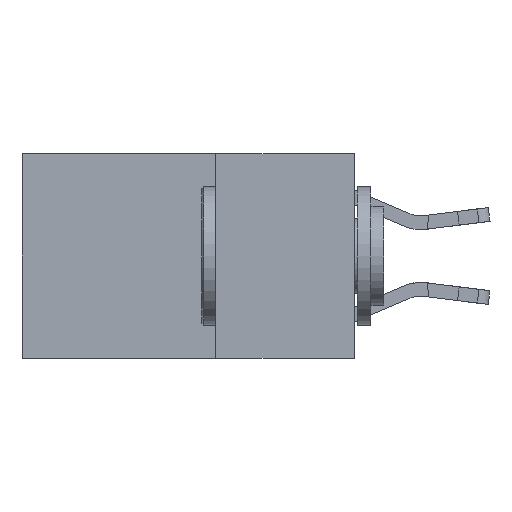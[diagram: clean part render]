
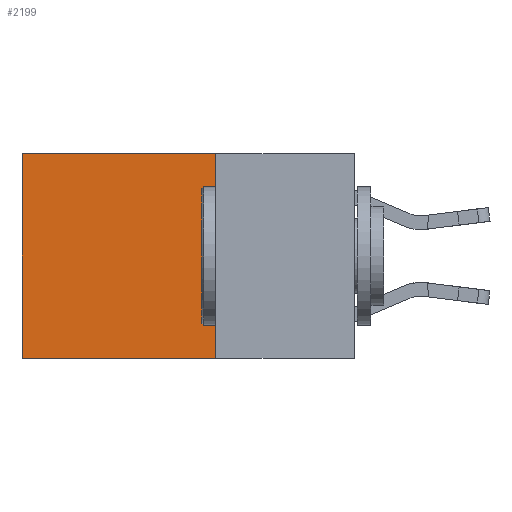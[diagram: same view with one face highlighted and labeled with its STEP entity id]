
A CAD part, left-side view. The second image highlights one B-rep face of the part: STEP entity #2199.
In plain terms, the highlighted planar face has unit normal (-1, 0, 0).
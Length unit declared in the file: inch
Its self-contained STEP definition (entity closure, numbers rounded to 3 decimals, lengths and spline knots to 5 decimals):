
#959 = LINE ( 'NONE', #7559, #9255 ) ;
#967 = EDGE_CURVE ( 'NONE', #9129, #4024, #16546, .T. ) ;
#1625 = VECTOR ( 'NONE', #23283, 39.37008 ) ;
#2199 = ADVANCED_FACE ( 'NONE', ( #18424 ), #14117, .F. ) ;
#2841 = CARTESIAN_POINT ( 'NONE',  ( 0.2625, 0.6, 0. ) ) ;
#4024 = VERTEX_POINT ( 'NONE', #13854 ) ;
#6850 = ORIENTED_EDGE ( 'NONE', *, *, #14675, .T. ) ;
#7559 = CARTESIAN_POINT ( 'NONE',  ( 0.2625, 0.6, 0. ) ) ;
#8101 = VERTEX_POINT ( 'NONE', #17261 ) ;
#9000 = CARTESIAN_POINT ( 'NONE',  ( 0.2625, 0.25, 0. ) ) ;
#9129 = VERTEX_POINT ( 'NONE', #9000 ) ;
#9190 = VERTEX_POINT ( 'NONE', #2841 ) ;
#9255 = VECTOR ( 'NONE', #14155, 39.37008 ) ;
#9317 = EDGE_CURVE ( 'NONE', #9190, #8101, #959, .T. ) ;
#9806 = DIRECTION ( 'NONE',  ( 0., 0., -1. ) ) ;
#10525 = DIRECTION ( 'NONE',  ( 0., 1., 0. ) ) ;
#12370 = ORIENTED_EDGE ( 'NONE', *, *, #967, .F. ) ;
#12374 = ORIENTED_EDGE ( 'NONE', *, *, #24601, .F. ) ;
#13854 = CARTESIAN_POINT ( 'NONE',  ( 0.2625, 0.25, -0.37 ) ) ;
#13942 = CARTESIAN_POINT ( 'NONE',  ( 0.2625, 0.25, -0.37 ) ) ;
#14117 = PLANE ( 'NONE',  #14273 ) ;
#14155 = DIRECTION ( 'NONE',  ( 0., 0., -1. ) ) ;
#14273 = AXIS2_PLACEMENT_3D ( 'NONE', #26725, #18560, #9806 ) ;
#14675 = EDGE_CURVE ( 'NONE', #9129, #9190, #19425, .T. ) ;
#14687 = CARTESIAN_POINT ( 'NONE',  ( 0.2625, 0.25, 0. ) ) ;
#16546 = LINE ( 'NONE', #14687, #1625 ) ;
#16808 = VECTOR ( 'NONE', #10525, 39.37008 ) ;
#17251 = ORIENTED_EDGE ( 'NONE', *, *, #9317, .T. ) ;
#17261 = CARTESIAN_POINT ( 'NONE',  ( 0.2625, 0.6, -0.37 ) ) ;
#18424 = FACE_OUTER_BOUND ( 'NONE', #27170, .T. ) ;
#18560 = DIRECTION ( 'NONE',  ( 1., 0., 0. ) ) ;
#19287 = CARTESIAN_POINT ( 'NONE',  ( 0.2625, 0.25, 0. ) ) ;
#19425 = LINE ( 'NONE', #19287, #16808 ) ;
#20512 = VECTOR ( 'NONE', #22535, 39.37008 ) ;
#20520 = LINE ( 'NONE', #13942, #20512 ) ;
#22535 = DIRECTION ( 'NONE',  ( 0., 1., 0. ) ) ;
#23283 = DIRECTION ( 'NONE',  ( 0., 0., -1. ) ) ;
#24601 = EDGE_CURVE ( 'NONE', #4024, #8101, #20520, .T. ) ;
#26725 = CARTESIAN_POINT ( 'NONE',  ( 0.2625, 0.25, 0. ) ) ;
#27170 = EDGE_LOOP ( 'NONE', ( #17251, #12374, #12370, #6850 ) ) ;
